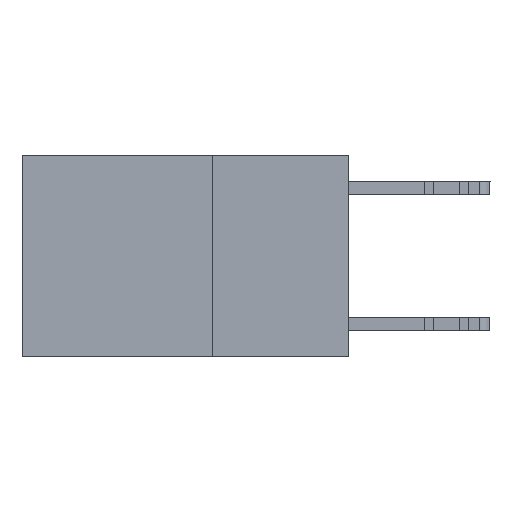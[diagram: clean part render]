
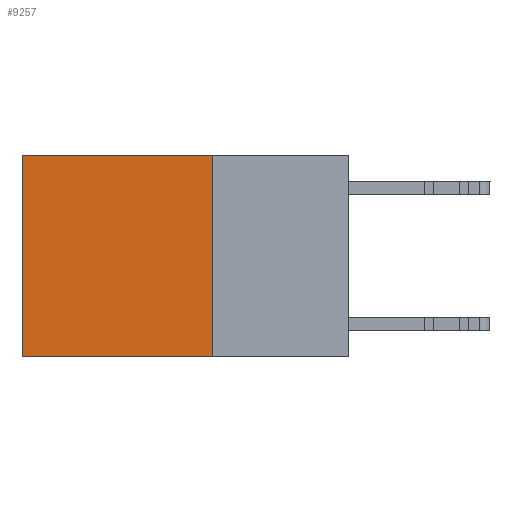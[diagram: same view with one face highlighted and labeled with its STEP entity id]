
A CAD part, left-side view. The second image highlights one B-rep face of the part: STEP entity #9257.
In plain terms, the highlighted planar face has unit normal (-1, 0, 0).
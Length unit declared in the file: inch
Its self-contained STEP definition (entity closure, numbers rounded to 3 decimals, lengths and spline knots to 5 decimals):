
#376 = DIRECTION ( 'NONE',  ( 1., 0., 0. ) ) ;
#503 = EDGE_CURVE ( 'NONE', #1908, #23247, #6225, .T. ) ;
#806 = CARTESIAN_POINT ( 'NONE',  ( 0.2625, 0.6, -0.37 ) ) ;
#1185 = DIRECTION ( 'NONE',  ( 0., 1., 0. ) ) ;
#1908 = VERTEX_POINT ( 'NONE', #15892 ) ;
#1977 = DIRECTION ( 'NONE',  ( 0., 0., -1. ) ) ;
#3757 = DIRECTION ( 'NONE',  ( 0., 0., -1. ) ) ;
#5805 = CARTESIAN_POINT ( 'NONE',  ( 0.2625, 0.6, 0. ) ) ;
#6225 = LINE ( 'NONE', #8947, #14241 ) ;
#8947 = CARTESIAN_POINT ( 'NONE',  ( 0.2625, 0.25, 0. ) ) ;
#9257 = ADVANCED_FACE ( 'NONE', ( #20947 ), #23371, .F. ) ;
#9460 = EDGE_CURVE ( 'NONE', #1908, #21984, #17446, .T. ) ;
#9640 = DIRECTION ( 'NONE',  ( 0., 0., -1. ) ) ;
#9662 = ORIENTED_EDGE ( 'NONE', *, *, #15886, .F. ) ;
#11107 = EDGE_LOOP ( 'NONE', ( #15166, #9662, #26002, #17283 ) ) ;
#12028 = CARTESIAN_POINT ( 'NONE',  ( 0.2625, 0.25, -0.37 ) ) ;
#14241 = VECTOR ( 'NONE', #1977, 39.37008 ) ;
#14301 = CARTESIAN_POINT ( 'NONE',  ( 0.2625, 0.25, 0. ) ) ;
#15166 = ORIENTED_EDGE ( 'NONE', *, *, #15848, .T. ) ;
#15848 = EDGE_CURVE ( 'NONE', #21984, #22027, #26732, .T. ) ;
#15886 = EDGE_CURVE ( 'NONE', #23247, #22027, #20227, .T. ) ;
#15892 = CARTESIAN_POINT ( 'NONE',  ( 0.2625, 0.25, 0. ) ) ;
#16988 = VECTOR ( 'NONE', #3757, 39.37008 ) ;
#17266 = VECTOR ( 'NONE', #26678, 39.37008 ) ;
#17283 = ORIENTED_EDGE ( 'NONE', *, *, #9460, .T. ) ;
#17446 = LINE ( 'NONE', #28964, #17266 ) ;
#20227 = LINE ( 'NONE', #24758, #25696 ) ;
#20947 = FACE_OUTER_BOUND ( 'NONE', #11107, .T. ) ;
#21984 = VERTEX_POINT ( 'NONE', #5805 ) ;
#22027 = VERTEX_POINT ( 'NONE', #806 ) ;
#23247 = VERTEX_POINT ( 'NONE', #12028 ) ;
#23371 = PLANE ( 'NONE',  #29355 ) ;
#24758 = CARTESIAN_POINT ( 'NONE',  ( 0.2625, 0.25, -0.37 ) ) ;
#25696 = VECTOR ( 'NONE', #1185, 39.37008 ) ;
#26002 = ORIENTED_EDGE ( 'NONE', *, *, #503, .F. ) ;
#26678 = DIRECTION ( 'NONE',  ( 0., 1., 0. ) ) ;
#26732 = LINE ( 'NONE', #29021, #16988 ) ;
#28964 = CARTESIAN_POINT ( 'NONE',  ( 0.2625, 0.25, 0. ) ) ;
#29021 = CARTESIAN_POINT ( 'NONE',  ( 0.2625, 0.6, 0. ) ) ;
#29355 = AXIS2_PLACEMENT_3D ( 'NONE', #14301, #376, #9640 ) ;
